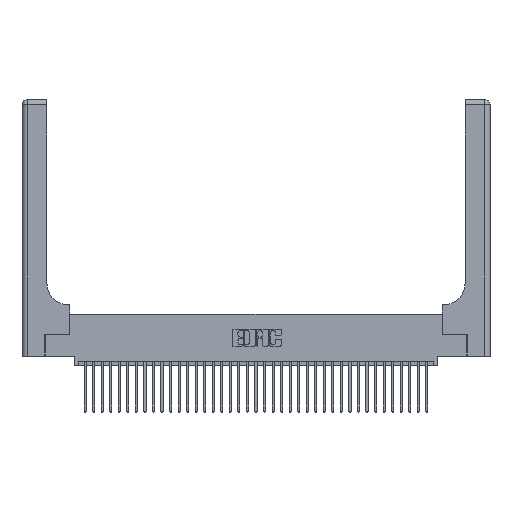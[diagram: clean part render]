
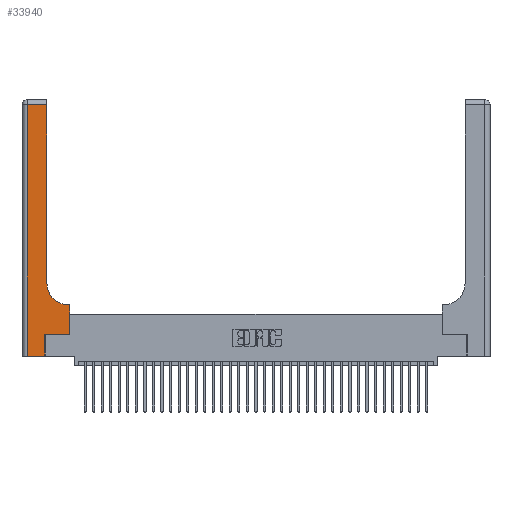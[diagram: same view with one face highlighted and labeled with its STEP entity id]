
A CAD part, top view. The second image highlights one B-rep face of the part: STEP entity #33940.
In plain terms, the highlighted planar face has unit normal (0, 0, 1).
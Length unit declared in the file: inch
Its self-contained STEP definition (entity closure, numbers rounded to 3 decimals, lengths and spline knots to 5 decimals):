
#109 = VERTEX_POINT ( 'NONE', #3312 ) ;
#1024 = LINE ( 'NONE', #9505, #31071 ) ;
#1120 = VERTEX_POINT ( 'NONE', #7962 ) ;
#1277 = ORIENTED_EDGE ( 'NONE', *, *, #13700, .T. ) ;
#2170 = CARTESIAN_POINT ( 'NONE',  ( 0.2915, 0.6, 0.37 ) ) ;
#2343 = LINE ( 'NONE', #37638, #24673 ) ;
#2804 = DIRECTION ( 'NONE',  ( 0., 1., 0. ) ) ;
#3312 = CARTESIAN_POINT ( 'NONE',  ( 0.06, 0., 0.37 ) ) ;
#3733 = AXIS2_PLACEMENT_3D ( 'NONE', #8996, #29364, #11896 ) ;
#3851 = EDGE_CURVE ( 'NONE', #27174, #30697, #21373, .T. ) ;
#5097 = DIRECTION ( 'NONE',  ( -1., 0., 0. ) ) ;
#5440 = DIRECTION ( 'NONE',  ( 0., 1., 0. ) ) ;
#6303 = EDGE_CURVE ( 'NONE', #1120, #25764, #32960, .T. ) ;
#6369 = EDGE_LOOP ( 'NONE', ( #23157, #30838, #24965, #27704, #1277, #25443, #18584, #35880, #21361 ) ) ;
#7962 = CARTESIAN_POINT ( 'NONE',  ( 0.5585, 0.6, 0.37 ) ) ;
#8996 = CARTESIAN_POINT ( 'NONE',  ( 0., 3., 0.37 ) ) ;
#9185 = EDGE_CURVE ( 'NONE', #25764, #36673, #28721, .T. ) ;
#9505 = CARTESIAN_POINT ( 'NONE',  ( 0.269, 0., 0.37 ) ) ;
#10130 = LINE ( 'NONE', #26130, #22940 ) ;
#10969 = EDGE_CURVE ( 'NONE', #34924, #1120, #14900, .T. ) ;
#11126 = CARTESIAN_POINT ( 'NONE',  ( 0.5585, 0.25, 0.37 ) ) ;
#11574 = VECTOR ( 'NONE', #5097, 39.37008 ) ;
#11896 = DIRECTION ( 'NONE',  ( -1., 0., 0. ) ) ;
#12924 = DIRECTION ( 'NONE',  ( 1., 0., 0. ) ) ;
#13150 = VERTEX_POINT ( 'NONE', #36165 ) ;
#13433 = VERTEX_POINT ( 'NONE', #34484 ) ;
#13489 = EDGE_CURVE ( 'NONE', #109, #13433, #10130, .T. ) ;
#13557 = CARTESIAN_POINT ( 'NONE',  ( 0.2915, 0.85, 0.37 ) ) ;
#13682 = CARTESIAN_POINT ( 'NONE',  ( 0.5415, 0.6, 0.37 ) ) ;
#13700 = EDGE_CURVE ( 'NONE', #13433, #13150, #1024, .T. ) ;
#13969 = VECTOR ( 'NONE', #5440, 39.37008 ) ;
#14731 = VECTOR ( 'NONE', #36104, 39.37008 ) ;
#14822 = CARTESIAN_POINT ( 'NONE',  ( 0.5415, 0.85, 0.37 ) ) ;
#14900 = LINE ( 'NONE', #11126, #13969 ) ;
#17642 = PLANE ( 'NONE',  #3733 ) ;
#17741 = DIRECTION ( 'NONE',  ( 1., 0., 0. ) ) ;
#18269 = VECTOR ( 'NONE', #12924, 39.37008 ) ;
#18584 = ORIENTED_EDGE ( 'NONE', *, *, #10969, .T. ) ;
#19714 = EDGE_CURVE ( 'NONE', #36673, #27174, #2343, .T. ) ;
#20464 = VECTOR ( 'NONE', #29856, 39.37008 ) ;
#21361 = ORIENTED_EDGE ( 'NONE', *, *, #9185, .T. ) ;
#21373 = LINE ( 'NONE', #27095, #20464 ) ;
#22321 = CARTESIAN_POINT ( 'NONE',  ( 0.06, 2.94, 0.37 ) ) ;
#22520 = LINE ( 'NONE', #30241, #14731 ) ;
#22940 = VECTOR ( 'NONE', #29032, 39.37008 ) ;
#23157 = ORIENTED_EDGE ( 'NONE', *, *, #19714, .T. ) ;
#23563 = FACE_OUTER_BOUND ( 'NONE', #6369, .T. ) ;
#24673 = VECTOR ( 'NONE', #2804, 39.37008 ) ;
#24680 = CARTESIAN_POINT ( 'NONE',  ( 0.269, 0.25, 0.37 ) ) ;
#24965 = ORIENTED_EDGE ( 'NONE', *, *, #36493, .T. ) ;
#25443 = ORIENTED_EDGE ( 'NONE', *, *, #25956, .T. ) ;
#25764 = VERTEX_POINT ( 'NONE', #13682 ) ;
#25956 = EDGE_CURVE ( 'NONE', #13150, #34924, #27865, .T. ) ;
#26130 = CARTESIAN_POINT ( 'NONE',  ( 0., 0., 0.37 ) ) ;
#26887 = CARTESIAN_POINT ( 'NONE',  ( 0.2915, 2.94, 0.37 ) ) ;
#27095 = CARTESIAN_POINT ( 'NONE',  ( 0., 2.94, 0.37 ) ) ;
#27174 = VERTEX_POINT ( 'NONE', #26887 ) ;
#27704 = ORIENTED_EDGE ( 'NONE', *, *, #13489, .T. ) ;
#27865 = LINE ( 'NONE', #24680, #18269 ) ;
#28721 = CIRCLE ( 'NONE', #30221, 0.25 ) ;
#29032 = DIRECTION ( 'NONE',  ( 1., 0., 0. ) ) ;
#29364 = DIRECTION ( 'NONE',  ( 0., 0., -1. ) ) ;
#29856 = DIRECTION ( 'NONE',  ( -1., 0., 0. ) ) ;
#29895 = DIRECTION ( 'NONE',  ( 0., 1., 0. ) ) ;
#30221 = AXIS2_PLACEMENT_3D ( 'NONE', #14822, #35167, #17741 ) ;
#30241 = CARTESIAN_POINT ( 'NONE',  ( 0.06, 3., 0.37 ) ) ;
#30697 = VERTEX_POINT ( 'NONE', #22321 ) ;
#30838 = ORIENTED_EDGE ( 'NONE', *, *, #3851, .T. ) ;
#31071 = VECTOR ( 'NONE', #29895, 39.37008 ) ;
#32960 = LINE ( 'NONE', #2170, #11574 ) ;
#33940 = ADVANCED_FACE ( 'NONE', ( #23563 ), #17642, .F. ) ;
#34484 = CARTESIAN_POINT ( 'NONE',  ( 0.269, 0., 0.37 ) ) ;
#34924 = VERTEX_POINT ( 'NONE', #37339 ) ;
#35167 = DIRECTION ( 'NONE',  ( 0., 0., -1. ) ) ;
#35880 = ORIENTED_EDGE ( 'NONE', *, *, #6303, .T. ) ;
#36104 = DIRECTION ( 'NONE',  ( 0., -1., 0. ) ) ;
#36165 = CARTESIAN_POINT ( 'NONE',  ( 0.269, 0.25, 0.37 ) ) ;
#36493 = EDGE_CURVE ( 'NONE', #30697, #109, #22520, .T. ) ;
#36673 = VERTEX_POINT ( 'NONE', #13557 ) ;
#37339 = CARTESIAN_POINT ( 'NONE',  ( 0.5585, 0.25, 0.37 ) ) ;
#37638 = CARTESIAN_POINT ( 'NONE',  ( 0.2915, 3., 0.37 ) ) ;
